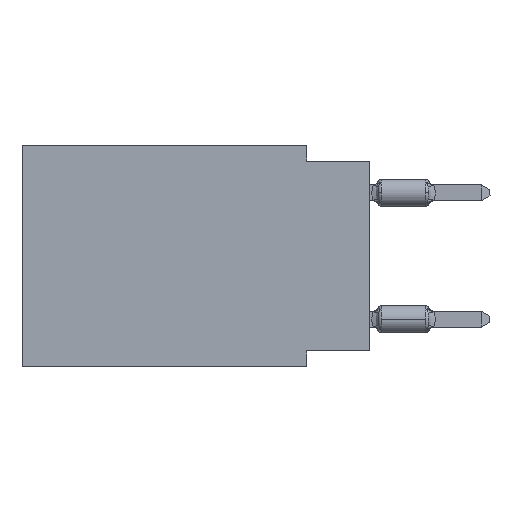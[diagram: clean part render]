
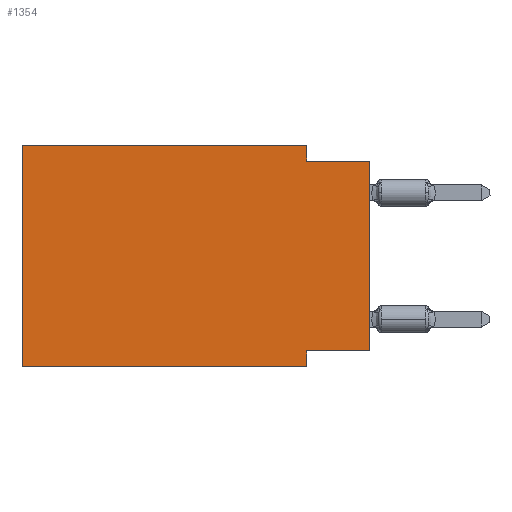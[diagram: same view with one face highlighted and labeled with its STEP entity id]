
A CAD part, left-side view. The second image highlights one B-rep face of the part: STEP entity #1354.
In plain terms, the highlighted planar face has unit normal (-1, 0, 0).
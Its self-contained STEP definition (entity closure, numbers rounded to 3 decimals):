
#361 = DIRECTION ( 'NONE',  ( 0., 0., 1. ) ) ;
#401 = DIRECTION ( 'NONE',  ( 0., 1., 0. ) ) ;
#424 = CARTESIAN_POINT ( 'NONE',  ( 0., 13.97, 0. ) ) ;
#567 = DIRECTION ( 'NONE',  ( 0., 0., 1. ) ) ;
#1314 = ORIENTED_EDGE ( 'NONE', *, *, #5642, .F. ) ;
#1354 = ADVANCED_FACE ( 'NONE', ( #4662 ), #5983, .F. ) ;
#1481 = EDGE_CURVE ( 'NONE', #4124, #4604, #11333, .T. ) ;
#1772 = CARTESIAN_POINT ( 'NONE',  ( 0., 0., 0. ) ) ;
#1904 = LINE ( 'NONE', #2003, #17837 ) ;
#2003 = CARTESIAN_POINT ( 'NONE',  ( 0., 0., -0.635 ) ) ;
#2021 = LINE ( 'NONE', #6253, #6877 ) ;
#2915 = CARTESIAN_POINT ( 'NONE',  ( 0., 13.97, -8.89 ) ) ;
#3324 = CARTESIAN_POINT ( 'NONE',  ( 0., 2.54, -8.255 ) ) ;
#3506 = DIRECTION ( 'NONE',  ( 0., 0., -1. ) ) ;
#4040 = CARTESIAN_POINT ( 'NONE',  ( 0., 0., -0.635 ) ) ;
#4124 = VERTEX_POINT ( 'NONE', #10687 ) ;
#4604 = VERTEX_POINT ( 'NONE', #9337 ) ;
#4662 = FACE_OUTER_BOUND ( 'NONE', #12401, .T. ) ;
#4821 = VERTEX_POINT ( 'NONE', #14955 ) ;
#4833 = ORIENTED_EDGE ( 'NONE', *, *, #5140, .T. ) ;
#5097 = VERTEX_POINT ( 'NONE', #17547 ) ;
#5140 = EDGE_CURVE ( 'NONE', #9019, #4821, #18354, .T. ) ;
#5642 = EDGE_CURVE ( 'NONE', #18950, #4821, #10463, .T. ) ;
#5983 = PLANE ( 'NONE',  #17316 ) ;
#6253 = CARTESIAN_POINT ( 'NONE',  ( 0., 0., -8.255 ) ) ;
#6282 = DIRECTION ( 'NONE',  ( 0., 0., -1. ) ) ;
#6877 = VECTOR ( 'NONE', #401, 1000. ) ;
#7806 = DIRECTION ( 'NONE',  ( 1., 0., 0. ) ) ;
#8166 = DIRECTION ( 'NONE',  ( 0., -1., 0. ) ) ;
#8262 = VECTOR ( 'NONE', #3506, 1000. ) ;
#8765 = ORIENTED_EDGE ( 'NONE', *, *, #18719, .T. ) ;
#9019 = VERTEX_POINT ( 'NONE', #12684 ) ;
#9197 = VERTEX_POINT ( 'NONE', #16489 ) ;
#9337 = CARTESIAN_POINT ( 'NONE',  ( 0., 2.54, 0. ) ) ;
#10162 = VECTOR ( 'NONE', #361, 1000. ) ;
#10463 = LINE ( 'NONE', #18126, #17225 ) ;
#10612 = EDGE_CURVE ( 'NONE', #9019, #4124, #15898, .T. ) ;
#10687 = CARTESIAN_POINT ( 'NONE',  ( 0., 13.97, 0. ) ) ;
#10845 = ORIENTED_EDGE ( 'NONE', *, *, #1481, .F. ) ;
#10964 = LINE ( 'NONE', #1772, #10162 ) ;
#11185 = LINE ( 'NONE', #17330, #8262 ) ;
#11205 = VECTOR ( 'NONE', #15961, 1000. ) ;
#11228 = VECTOR ( 'NONE', #567, 1000. ) ;
#11333 = LINE ( 'NONE', #424, #11205 ) ;
#12149 = CARTESIAN_POINT ( 'NONE',  ( 0., 13.97, 0. ) ) ;
#12401 = EDGE_LOOP ( 'NONE', ( #8765, #19694, #12923, #10845, #16236, #4833, #1314, #14651 ) ) ;
#12684 = CARTESIAN_POINT ( 'NONE',  ( 0., 13.97, -8.89 ) ) ;
#12923 = ORIENTED_EDGE ( 'NONE', *, *, #19572, .F. ) ;
#13729 = DIRECTION ( 'NONE',  ( 0., -1., 0. ) ) ;
#14046 = VERTEX_POINT ( 'NONE', #4040 ) ;
#14407 = CARTESIAN_POINT ( 'NONE',  ( 0., 13.97, 0. ) ) ;
#14651 = ORIENTED_EDGE ( 'NONE', *, *, #16355, .F. ) ;
#14955 = CARTESIAN_POINT ( 'NONE',  ( 0., 2.54, -8.89 ) ) ;
#15898 = LINE ( 'NONE', #14407, #11228 ) ;
#15935 = VECTOR ( 'NONE', #13729, 1000. ) ;
#15961 = DIRECTION ( 'NONE',  ( 0., -1., 0. ) ) ;
#16236 = ORIENTED_EDGE ( 'NONE', *, *, #10612, .F. ) ;
#16355 = EDGE_CURVE ( 'NONE', #5097, #18950, #2021, .T. ) ;
#16489 = CARTESIAN_POINT ( 'NONE',  ( 0., 2.54, -0.635 ) ) ;
#17225 = VECTOR ( 'NONE', #17820, 1000. ) ;
#17316 = AXIS2_PLACEMENT_3D ( 'NONE', #12149, #7806, #6282 ) ;
#17330 = CARTESIAN_POINT ( 'NONE',  ( 0., 2.54, 0. ) ) ;
#17547 = CARTESIAN_POINT ( 'NONE',  ( 0., 0., -8.255 ) ) ;
#17820 = DIRECTION ( 'NONE',  ( 0., 0., -1. ) ) ;
#17837 = VECTOR ( 'NONE', #8166, 1000. ) ;
#17995 = EDGE_CURVE ( 'NONE', #9197, #14046, #1904, .T. ) ;
#18126 = CARTESIAN_POINT ( 'NONE',  ( 0., 2.54, -8.89 ) ) ;
#18354 = LINE ( 'NONE', #2915, #15935 ) ;
#18719 = EDGE_CURVE ( 'NONE', #5097, #14046, #10964, .T. ) ;
#18950 = VERTEX_POINT ( 'NONE', #3324 ) ;
#19572 = EDGE_CURVE ( 'NONE', #4604, #9197, #11185, .T. ) ;
#19694 = ORIENTED_EDGE ( 'NONE', *, *, #17995, .F. ) ;
